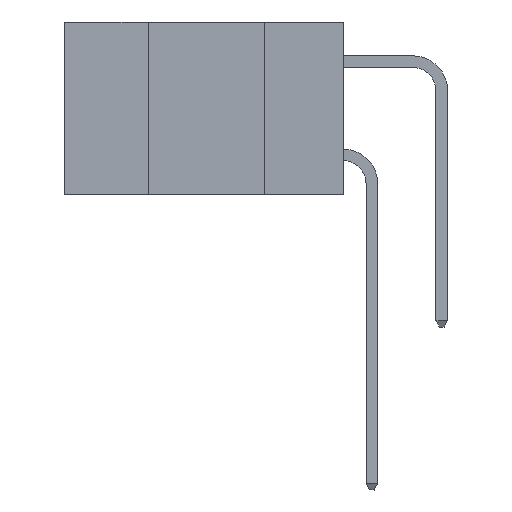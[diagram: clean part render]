
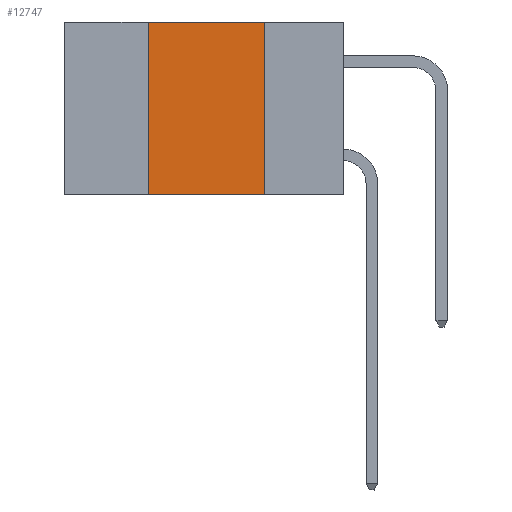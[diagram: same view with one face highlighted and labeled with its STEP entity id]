
A CAD part, left-side view. The second image highlights one B-rep face of the part: STEP entity #12747.
In plain terms, the highlighted planar face has unit normal (-1, 0, 0).
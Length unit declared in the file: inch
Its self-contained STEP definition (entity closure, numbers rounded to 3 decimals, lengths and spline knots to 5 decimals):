
#117 = CARTESIAN_POINT ( 'NONE',  ( 0., 0.42, -0.37 ) ) ;
#127 = CARTESIAN_POINT ( 'NONE',  ( 0., 0.17, 0. ) ) ;
#155 = LINE ( 'NONE', #2072, #5753 ) ;
#2072 = CARTESIAN_POINT ( 'NONE',  ( 0., 0.17, 0. ) ) ;
#2515 = VERTEX_POINT ( 'NONE', #127 ) ;
#3254 = DIRECTION ( 'NONE',  ( 1., 0., 0. ) ) ;
#3756 = ORIENTED_EDGE ( 'NONE', *, *, #16414, .T. ) ;
#3951 = EDGE_CURVE ( 'NONE', #2515, #14508, #155, .T. ) ;
#4811 = DIRECTION ( 'NONE',  ( 0., 0., -1. ) ) ;
#5191 = VECTOR ( 'NONE', #19098, 39.37008 ) ;
#5753 = VECTOR ( 'NONE', #19264, 39.37008 ) ;
#5775 = VECTOR ( 'NONE', #12591, 39.37008 ) ;
#5948 = EDGE_CURVE ( 'NONE', #16619, #2515, #16167, .T. ) ;
#6674 = DIRECTION ( 'NONE',  ( 0., 0., 1. ) ) ;
#8961 = VERTEX_POINT ( 'NONE', #117 ) ;
#10658 = LINE ( 'NONE', #18137, #5775 ) ;
#10758 = ORIENTED_EDGE ( 'NONE', *, *, #5948, .F. ) ;
#11123 = PLANE ( 'NONE',  #15326 ) ;
#12315 = ORIENTED_EDGE ( 'NONE', *, *, #3951, .F. ) ;
#12350 = ORIENTED_EDGE ( 'NONE', *, *, #18033, .F. ) ;
#12480 = LINE ( 'NONE', #19366, #14387 ) ;
#12591 = DIRECTION ( 'NONE',  ( 0., -1., 0. ) ) ;
#12747 = ADVANCED_FACE ( 'NONE', ( #14645 ), #11123, .F. ) ;
#14387 = VECTOR ( 'NONE', #6674, 39.37008 ) ;
#14508 = VERTEX_POINT ( 'NONE', #15576 ) ;
#14645 = FACE_OUTER_BOUND ( 'NONE', #20142, .T. ) ;
#15326 = AXIS2_PLACEMENT_3D ( 'NONE', #15783, #3254, #4811 ) ;
#15576 = CARTESIAN_POINT ( 'NONE',  ( 0., 0.17, -0.37 ) ) ;
#15783 = CARTESIAN_POINT ( 'NONE',  ( 0., 0.6, 0. ) ) ;
#16167 = LINE ( 'NONE', #17638, #5191 ) ;
#16414 = EDGE_CURVE ( 'NONE', #8961, #14508, #10658, .T. ) ;
#16619 = VERTEX_POINT ( 'NONE', #16816 ) ;
#16816 = CARTESIAN_POINT ( 'NONE',  ( 0., 0.42, 0. ) ) ;
#17638 = CARTESIAN_POINT ( 'NONE',  ( 0., 0.6, 0. ) ) ;
#18033 = EDGE_CURVE ( 'NONE', #8961, #16619, #12480, .T. ) ;
#18137 = CARTESIAN_POINT ( 'NONE',  ( 0., 0.6, -0.37 ) ) ;
#19098 = DIRECTION ( 'NONE',  ( 0., -1., 0. ) ) ;
#19264 = DIRECTION ( 'NONE',  ( 0., 0., -1. ) ) ;
#19366 = CARTESIAN_POINT ( 'NONE',  ( 0., 0.42, 0. ) ) ;
#20142 = EDGE_LOOP ( 'NONE', ( #12315, #10758, #12350, #3756 ) ) ;
